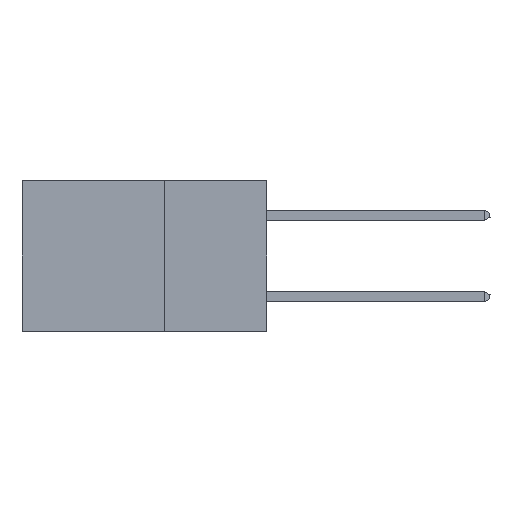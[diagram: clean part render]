
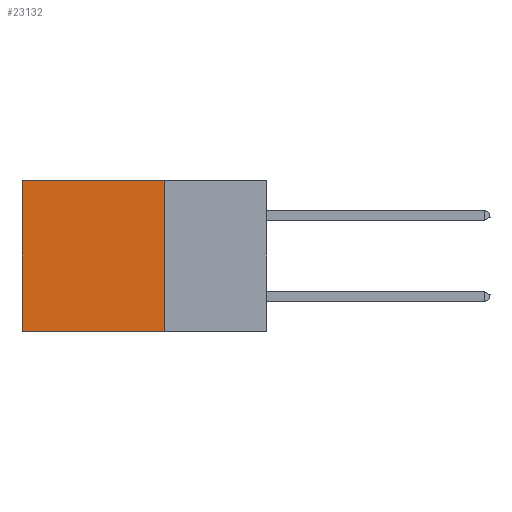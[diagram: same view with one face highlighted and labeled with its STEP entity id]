
A CAD part, left-side view. The second image highlights one B-rep face of the part: STEP entity #23132.
In plain terms, the highlighted planar face has unit normal (-1, 0, 0).
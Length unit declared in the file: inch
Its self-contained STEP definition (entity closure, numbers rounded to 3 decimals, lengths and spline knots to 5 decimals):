
#2675 = CARTESIAN_POINT ( 'NONE',  ( 0.2875, 0.25, 0. ) ) ;
#4238 = DIRECTION ( 'NONE',  ( 0., 1., 0. ) ) ;
#4405 = VECTOR ( 'NONE', #43413, 39.37008 ) ;
#5866 = EDGE_CURVE ( 'NONE', #15476, #38374, #12971, .T. ) ;
#7056 = ORIENTED_EDGE ( 'NONE', *, *, #21547, .F. ) ;
#7750 = EDGE_CURVE ( 'NONE', #19327, #31029, #14436, .T. ) ;
#7948 = DIRECTION ( 'NONE',  ( 0., 0., -1. ) ) ;
#9548 = ORIENTED_EDGE ( 'NONE', *, *, #7750, .T. ) ;
#12971 = LINE ( 'NONE', #2675, #4405 ) ;
#14073 = CARTESIAN_POINT ( 'NONE',  ( 0.2875, 0.6, -0.37 ) ) ;
#14436 = LINE ( 'NONE', #43574, #34037 ) ;
#14794 = CARTESIAN_POINT ( 'NONE',  ( 0.2875, 0.25, 0. ) ) ;
#15476 = VERTEX_POINT ( 'NONE', #24490 ) ;
#16139 = CARTESIAN_POINT ( 'NONE',  ( 0.2875, 0.6, 0. ) ) ;
#18232 = PLANE ( 'NONE',  #43235 ) ;
#19327 = VERTEX_POINT ( 'NONE', #16139 ) ;
#20812 = VECTOR ( 'NONE', #33741, 39.37008 ) ;
#21547 = EDGE_CURVE ( 'NONE', #38374, #31029, #28776, .T. ) ;
#22352 = EDGE_LOOP ( 'NONE', ( #9548, #7056, #23494, #41265 ) ) ;
#23132 = ADVANCED_FACE ( 'NONE', ( #31099 ), #18232, .F. ) ;
#23494 = ORIENTED_EDGE ( 'NONE', *, *, #5866, .F. ) ;
#23965 = CARTESIAN_POINT ( 'NONE',  ( 0.2875, 0.25, -0.37 ) ) ;
#24490 = CARTESIAN_POINT ( 'NONE',  ( 0.2875, 0.25, 0. ) ) ;
#26399 = VECTOR ( 'NONE', #4238, 39.37008 ) ;
#27701 = LINE ( 'NONE', #38265, #26399 ) ;
#28776 = LINE ( 'NONE', #23965, #20812 ) ;
#29452 = DIRECTION ( 'NONE',  ( 0., 0., -1. ) ) ;
#31029 = VERTEX_POINT ( 'NONE', #14073 ) ;
#31099 = FACE_OUTER_BOUND ( 'NONE', #22352, .T. ) ;
#31696 = DIRECTION ( 'NONE',  ( 1., 0., 0. ) ) ;
#33741 = DIRECTION ( 'NONE',  ( 0., 1., 0. ) ) ;
#34037 = VECTOR ( 'NONE', #29452, 39.37008 ) ;
#35447 = CARTESIAN_POINT ( 'NONE',  ( 0.2875, 0.25, -0.37 ) ) ;
#38265 = CARTESIAN_POINT ( 'NONE',  ( 0.2875, 0.25, 0. ) ) ;
#38374 = VERTEX_POINT ( 'NONE', #35447 ) ;
#41265 = ORIENTED_EDGE ( 'NONE', *, *, #41680, .T. ) ;
#41680 = EDGE_CURVE ( 'NONE', #15476, #19327, #27701, .T. ) ;
#43235 = AXIS2_PLACEMENT_3D ( 'NONE', #14794, #31696, #7948 ) ;
#43413 = DIRECTION ( 'NONE',  ( 0., 0., -1. ) ) ;
#43574 = CARTESIAN_POINT ( 'NONE',  ( 0.2875, 0.6, 0. ) ) ;
